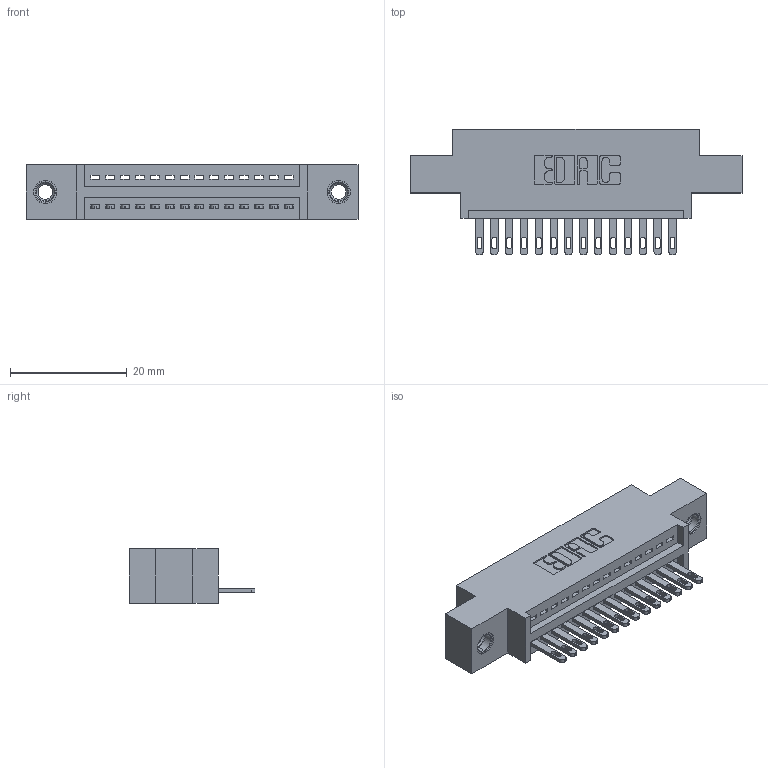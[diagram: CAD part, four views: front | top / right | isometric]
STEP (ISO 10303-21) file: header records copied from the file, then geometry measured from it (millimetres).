
FILE_DESCRIPTION (( 'STEP AP203' ), '1' );
FILE_NAME ('895-014-500-607.STEP', '2020-09-25T03:02:10', ( '' ), ( '' ), 'SwSTEP 2.0', 'SolidWorks 2020', '' );
FILE_SCHEMA (( 'CONFIG_CONTROL_DESIGN' ));
Length unit declared in the file: inch
Products named in the file (4): 345-292-001_345-293-100; 345-250-001_345-250-005-103; 845 Part_0.170 Offset - 0.156 Dia-TI; 895-014-500-607
Assembly tree (17 placements, depth 2):
  895-014-500-607
    845 Part_0.170 Offset - 0.156 Dia-TI
    345-292-001_345-293-100  x14
    345-250-001_345-250-005-103  x2
Bounding box: 56.77 x 21.51 x 9.4 mm (x, y, z)
Volume: 5044.4 mm3; surface area: 6513.5 mm2
Topology: 17 solids, 17 shells, 946 faces, 2841 edges, 1886 vertices
Faces by surface type: plane 592, cylinder 338, cone 12, torus 4
Entity records: 15554 total; most frequent: CARTESIAN_POINT 2677, ORIENTED_EDGE 2618, DIRECTION 2407, EDGE_CURVE 1309, LINE 1097, VECTOR 1097, VERTEX_POINT 868, AXIS2_PLACEMENT_3D 655
